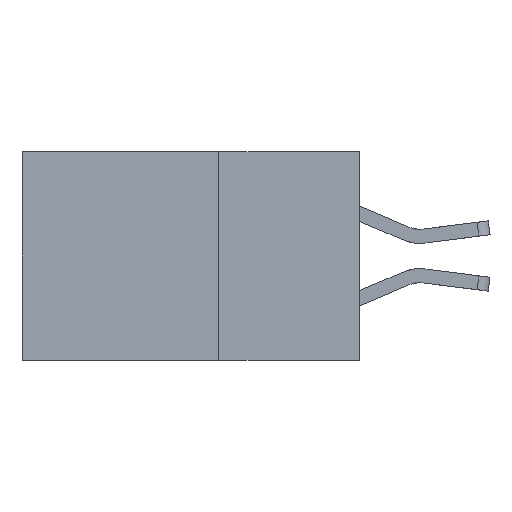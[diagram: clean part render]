
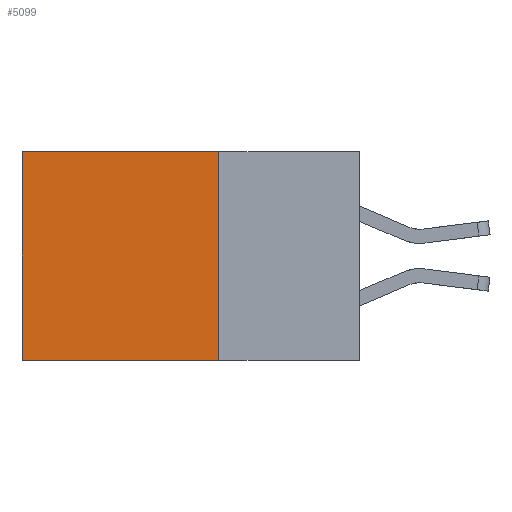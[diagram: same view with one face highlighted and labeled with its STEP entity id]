
A CAD part, left-side view. The second image highlights one B-rep face of the part: STEP entity #5099.
In plain terms, the highlighted planar face has unit normal (-1, 0, 0).
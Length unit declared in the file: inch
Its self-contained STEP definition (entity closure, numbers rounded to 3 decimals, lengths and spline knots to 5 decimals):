
#108 = DIRECTION ( 'NONE',  ( 0., 1., 0. ) ) ;
#392 = AXIS2_PLACEMENT_3D ( 'NONE', #12054, #4571, #12294 ) ;
#401 = VERTEX_POINT ( 'NONE', #5324 ) ;
#2504 = LINE ( 'NONE', #3411, #5031 ) ;
#2634 = VERTEX_POINT ( 'NONE', #11161 ) ;
#2648 = EDGE_LOOP ( 'NONE', ( #11210, #10817, #11397, #11939 ) ) ;
#2736 = VECTOR ( 'NONE', #5207, 39.37008 ) ;
#2864 = CARTESIAN_POINT ( 'NONE',  ( 0.2875, 0.25, -0.37 ) ) ;
#3411 = CARTESIAN_POINT ( 'NONE',  ( 0.2875, 0.25, 0. ) ) ;
#3438 = DIRECTION ( 'NONE',  ( 0., 1., 0. ) ) ;
#4286 = CARTESIAN_POINT ( 'NONE',  ( 0.2875, 0.25, 0. ) ) ;
#4309 = EDGE_CURVE ( 'NONE', #2634, #401, #2504, .T. ) ;
#4450 = FACE_OUTER_BOUND ( 'NONE', #2648, .T. ) ;
#4571 = DIRECTION ( 'NONE',  ( 1., 0., 0. ) ) ;
#5031 = VECTOR ( 'NONE', #11994, 39.37008 ) ;
#5045 = VERTEX_POINT ( 'NONE', #11037 ) ;
#5099 = ADVANCED_FACE ( 'NONE', ( #4450 ), #5356, .F. ) ;
#5207 = DIRECTION ( 'NONE',  ( 0., 0., -1. ) ) ;
#5271 = VECTOR ( 'NONE', #3438, 39.37008 ) ;
#5324 = CARTESIAN_POINT ( 'NONE',  ( 0.2875, 0.25, -0.37 ) ) ;
#5356 = PLANE ( 'NONE',  #392 ) ;
#6779 = CARTESIAN_POINT ( 'NONE',  ( 0.2875, 0.6, 0. ) ) ;
#7465 = EDGE_CURVE ( 'NONE', #2634, #10801, #9755, .T. ) ;
#8603 = LINE ( 'NONE', #2864, #10221 ) ;
#9755 = LINE ( 'NONE', #4286, #5271 ) ;
#10221 = VECTOR ( 'NONE', #108, 39.37008 ) ;
#10797 = LINE ( 'NONE', #10857, #2736 ) ;
#10801 = VERTEX_POINT ( 'NONE', #6779 ) ;
#10817 = ORIENTED_EDGE ( 'NONE', *, *, #12093, .F. ) ;
#10857 = CARTESIAN_POINT ( 'NONE',  ( 0.2875, 0.6, 0. ) ) ;
#11037 = CARTESIAN_POINT ( 'NONE',  ( 0.2875, 0.6, -0.37 ) ) ;
#11161 = CARTESIAN_POINT ( 'NONE',  ( 0.2875, 0.25, 0. ) ) ;
#11210 = ORIENTED_EDGE ( 'NONE', *, *, #11691, .T. ) ;
#11397 = ORIENTED_EDGE ( 'NONE', *, *, #4309, .F. ) ;
#11691 = EDGE_CURVE ( 'NONE', #10801, #5045, #10797, .T. ) ;
#11939 = ORIENTED_EDGE ( 'NONE', *, *, #7465, .T. ) ;
#11994 = DIRECTION ( 'NONE',  ( 0., 0., -1. ) ) ;
#12054 = CARTESIAN_POINT ( 'NONE',  ( 0.2875, 0.25, 0. ) ) ;
#12093 = EDGE_CURVE ( 'NONE', #401, #5045, #8603, .T. ) ;
#12294 = DIRECTION ( 'NONE',  ( 0., 0., -1. ) ) ;
